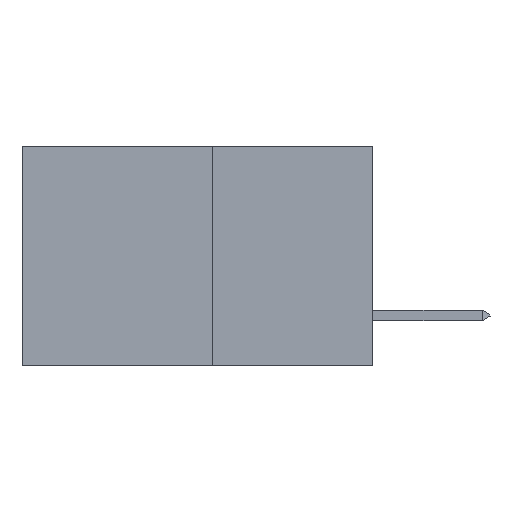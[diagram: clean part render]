
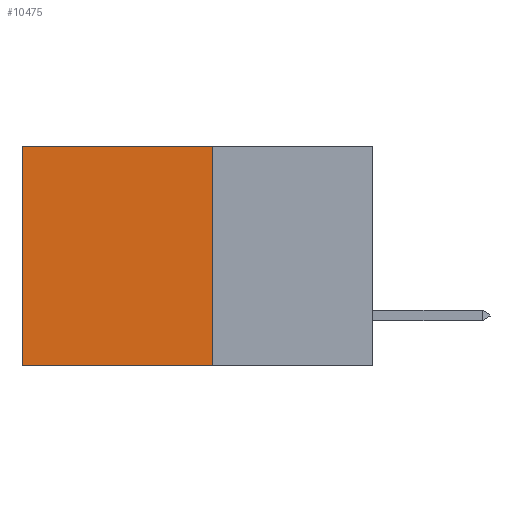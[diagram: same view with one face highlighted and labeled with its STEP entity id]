
A CAD part, left-side view. The second image highlights one B-rep face of the part: STEP entity #10475.
In plain terms, the highlighted planar face has unit normal (-1, 0, 0).
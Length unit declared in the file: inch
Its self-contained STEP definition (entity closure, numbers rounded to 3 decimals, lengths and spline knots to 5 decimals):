
#14 = CARTESIAN_POINT ( 'NONE',  ( 0.277, 0.59, -0.37 ) ) ;
#1440 = LINE ( 'NONE', #14, #16248 ) ;
#1582 = ORIENTED_EDGE ( 'NONE', *, *, #5931, .T. ) ;
#1610 = PLANE ( 'NONE',  #19156 ) ;
#2183 = VECTOR ( 'NONE', #7776, 39.37008 ) ;
#2242 = CARTESIAN_POINT ( 'NONE',  ( 0.277, 0.27, 0. ) ) ;
#3124 = DIRECTION ( 'NONE',  ( 1., 0., 0. ) ) ;
#3145 = EDGE_LOOP ( 'NONE', ( #16702, #15860, #4886, #1582 ) ) ;
#3938 = CARTESIAN_POINT ( 'NONE',  ( 0.277, 0.59, 0. ) ) ;
#4886 = ORIENTED_EDGE ( 'NONE', *, *, #7396, .F. ) ;
#5931 = EDGE_CURVE ( 'NONE', #16050, #9088, #15665, .T. ) ;
#7396 = EDGE_CURVE ( 'NONE', #16050, #16305, #8127, .T. ) ;
#7776 = DIRECTION ( 'NONE',  ( 0., 1., 0. ) ) ;
#8127 = LINE ( 'NONE', #16181, #15382 ) ;
#8703 = FACE_OUTER_BOUND ( 'NONE', #3145, .T. ) ;
#9088 = VERTEX_POINT ( 'NONE', #3938 ) ;
#9092 = CARTESIAN_POINT ( 'NONE',  ( 0.277, 0.27, -0.37 ) ) ;
#10457 = VECTOR ( 'NONE', #11215, 39.37008 ) ;
#10475 = ADVANCED_FACE ( 'NONE', ( #8703 ), #1610, .F. ) ;
#10599 = CARTESIAN_POINT ( 'NONE',  ( 0.277, 0.27, -0.37 ) ) ;
#11215 = DIRECTION ( 'NONE',  ( 0., 1., 0. ) ) ;
#13489 = DIRECTION ( 'NONE',  ( 0., 0., -1. ) ) ;
#13562 = LINE ( 'NONE', #17857, #2183 ) ;
#15382 = VECTOR ( 'NONE', #17583, 39.37008 ) ;
#15665 = LINE ( 'NONE', #2242, #10457 ) ;
#15701 = EDGE_CURVE ( 'NONE', #16305, #17655, #13562, .T. ) ;
#15860 = ORIENTED_EDGE ( 'NONE', *, *, #15701, .F. ) ;
#16050 = VERTEX_POINT ( 'NONE', #17417 ) ;
#16181 = CARTESIAN_POINT ( 'NONE',  ( 0.277, 0.27, -0.37 ) ) ;
#16248 = VECTOR ( 'NONE', #17476, 39.37008 ) ;
#16305 = VERTEX_POINT ( 'NONE', #9092 ) ;
#16702 = ORIENTED_EDGE ( 'NONE', *, *, #17473, .T. ) ;
#16737 = CARTESIAN_POINT ( 'NONE',  ( 0.277, 0.59, -0.37 ) ) ;
#17417 = CARTESIAN_POINT ( 'NONE',  ( 0.277, 0.27, 0. ) ) ;
#17473 = EDGE_CURVE ( 'NONE', #9088, #17655, #1440, .T. ) ;
#17476 = DIRECTION ( 'NONE',  ( 0., 0., -1. ) ) ;
#17583 = DIRECTION ( 'NONE',  ( 0., 0., -1. ) ) ;
#17655 = VERTEX_POINT ( 'NONE', #16737 ) ;
#17857 = CARTESIAN_POINT ( 'NONE',  ( 0.277, 0.27, -0.37 ) ) ;
#19156 = AXIS2_PLACEMENT_3D ( 'NONE', #10599, #3124, #13489 ) ;
